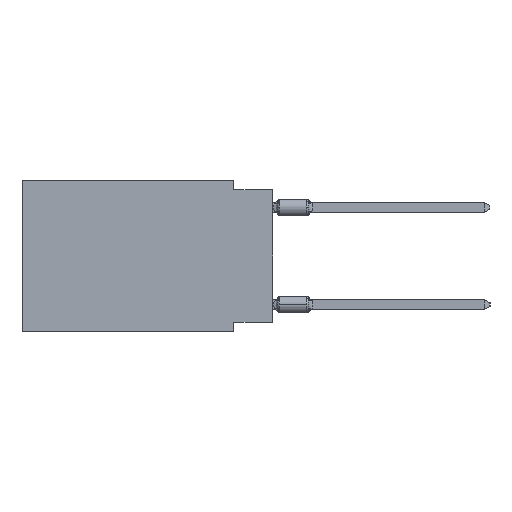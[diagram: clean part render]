
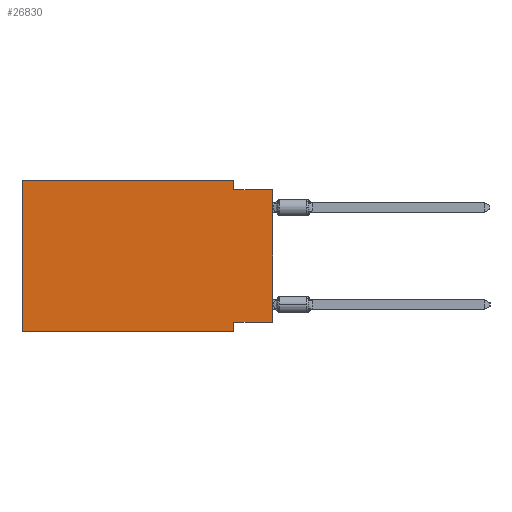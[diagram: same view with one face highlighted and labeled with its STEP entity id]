
A CAD part, left-side view. The second image highlights one B-rep face of the part: STEP entity #26830.
In plain terms, the highlighted planar face has unit normal (-1, 0, 0).
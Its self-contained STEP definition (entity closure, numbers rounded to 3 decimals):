
#1656 = VERTEX_POINT ( 'NONE', #13476 ) ;
#2835 = EDGE_CURVE ( 'NONE', #36846, #53293, #36777, .T. ) ;
#3294 = LINE ( 'NONE', #22008, #25750 ) ;
#3314 = EDGE_CURVE ( 'NONE', #1656, #3857, #3294, .T. ) ;
#3857 = VERTEX_POINT ( 'NONE', #24038 ) ;
#5793 = VECTOR ( 'NONE', #22888, 1000. ) ;
#7104 = VECTOR ( 'NONE', #51189, 1000. ) ;
#7922 = PLANE ( 'NONE',  #25090 ) ;
#9522 = CARTESIAN_POINT ( 'NONE',  ( 0., 16.383, -9.906 ) ) ;
#9860 = CARTESIAN_POINT ( 'NONE',  ( 0., 0., -0.635 ) ) ;
#9991 = ORIENTED_EDGE ( 'NONE', *, *, #3314, .F. ) ;
#10220 = LINE ( 'NONE', #24610, #37928 ) ;
#10678 = CARTESIAN_POINT ( 'NONE',  ( 0., 0., -0.635 ) ) ;
#13476 = CARTESIAN_POINT ( 'NONE',  ( 0., 2.54, 0. ) ) ;
#14416 = ORIENTED_EDGE ( 'NONE', *, *, #55931, .T. ) ;
#14498 = EDGE_CURVE ( 'NONE', #38452, #37792, #14931, .T. ) ;
#14931 = LINE ( 'NONE', #28710, #5793 ) ;
#15422 = CARTESIAN_POINT ( 'NONE',  ( 0., 16.383, 0. ) ) ;
#17288 = DIRECTION ( 'NONE',  ( 0., -1., 0. ) ) ;
#17374 = EDGE_CURVE ( 'NONE', #3857, #59659, #52389, .T. ) ;
#22008 = CARTESIAN_POINT ( 'NONE',  ( 0., 2.54, 0. ) ) ;
#22171 = ORIENTED_EDGE ( 'NONE', *, *, #48572, .F. ) ;
#22303 = DIRECTION ( 'NONE',  ( 0., 0., -1. ) ) ;
#22888 = DIRECTION ( 'NONE',  ( 0., 1., 0. ) ) ;
#24038 = CARTESIAN_POINT ( 'NONE',  ( 0., 2.54, -0.635 ) ) ;
#24314 = DIRECTION ( 'NONE',  ( 0., 0., 1. ) ) ;
#24610 = CARTESIAN_POINT ( 'NONE',  ( 0., 0., 0. ) ) ;
#25090 = AXIS2_PLACEMENT_3D ( 'NONE', #15422, #57725, #45037 ) ;
#25750 = VECTOR ( 'NONE', #22303, 1000. ) ;
#26473 = CARTESIAN_POINT ( 'NONE',  ( 0., 16.383, 0. ) ) ;
#26830 = ADVANCED_FACE ( 'NONE', ( #48516 ), #7922, .F. ) ;
#28158 = CARTESIAN_POINT ( 'NONE',  ( 0., 0., -9.271 ) ) ;
#28364 = VECTOR ( 'NONE', #52691, 1000. ) ;
#28621 = VECTOR ( 'NONE', #36361, 1000. ) ;
#28710 = CARTESIAN_POINT ( 'NONE',  ( 0., 0., -9.271 ) ) ;
#30151 = ORIENTED_EDGE ( 'NONE', *, *, #17374, .F. ) ;
#30819 = ORIENTED_EDGE ( 'NONE', *, *, #2835, .F. ) ;
#31562 = CARTESIAN_POINT ( 'NONE',  ( 0., 16.383, 0. ) ) ;
#33515 = CARTESIAN_POINT ( 'NONE',  ( 0., 16.383, -9.906 ) ) ;
#33517 = VECTOR ( 'NONE', #17288, 1000. ) ;
#35246 = LINE ( 'NONE', #33515, #36042 ) ;
#36042 = VECTOR ( 'NONE', #57150, 1000. ) ;
#36065 = LINE ( 'NONE', #59680, #28621 ) ;
#36361 = DIRECTION ( 'NONE',  ( 0., 0., -1. ) ) ;
#36777 = LINE ( 'NONE', #31562, #7104 ) ;
#36846 = VERTEX_POINT ( 'NONE', #9522 ) ;
#37792 = VERTEX_POINT ( 'NONE', #58332 ) ;
#37928 = VECTOR ( 'NONE', #24314, 1000. ) ;
#38452 = VERTEX_POINT ( 'NONE', #28158 ) ;
#39020 = ORIENTED_EDGE ( 'NONE', *, *, #14498, .F. ) ;
#39367 = EDGE_CURVE ( 'NONE', #36846, #41513, #35246, .T. ) ;
#41513 = VERTEX_POINT ( 'NONE', #42693 ) ;
#41861 = ORIENTED_EDGE ( 'NONE', *, *, #39367, .T. ) ;
#42693 = CARTESIAN_POINT ( 'NONE',  ( 0., 2.54, -9.906 ) ) ;
#43896 = EDGE_CURVE ( 'NONE', #37792, #41513, #36065, .T. ) ;
#45037 = DIRECTION ( 'NONE',  ( 0., 0., -1. ) ) ;
#45483 = CARTESIAN_POINT ( 'NONE',  ( 0., 16.383, 0. ) ) ;
#48516 = FACE_OUTER_BOUND ( 'NONE', #48966, .T. ) ;
#48572 = EDGE_CURVE ( 'NONE', #53293, #1656, #54407, .T. ) ;
#48966 = EDGE_LOOP ( 'NONE', ( #14416, #30151, #9991, #22171, #30819, #41861, #55927, #39020 ) ) ;
#51189 = DIRECTION ( 'NONE',  ( 0., 0., 1. ) ) ;
#52389 = LINE ( 'NONE', #10678, #28364 ) ;
#52691 = DIRECTION ( 'NONE',  ( 0., -1., 0. ) ) ;
#53293 = VERTEX_POINT ( 'NONE', #45483 ) ;
#54407 = LINE ( 'NONE', #26473, #33517 ) ;
#55927 = ORIENTED_EDGE ( 'NONE', *, *, #43896, .F. ) ;
#55931 = EDGE_CURVE ( 'NONE', #38452, #59659, #10220, .T. ) ;
#57150 = DIRECTION ( 'NONE',  ( 0., -1., 0. ) ) ;
#57725 = DIRECTION ( 'NONE',  ( 1., 0., 0. ) ) ;
#58332 = CARTESIAN_POINT ( 'NONE',  ( 0., 2.54, -9.271 ) ) ;
#59659 = VERTEX_POINT ( 'NONE', #9860 ) ;
#59680 = CARTESIAN_POINT ( 'NONE',  ( 0., 2.54, -9.906 ) ) ;
